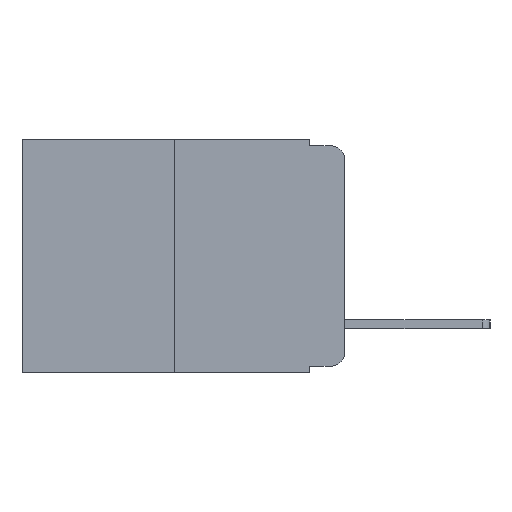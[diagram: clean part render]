
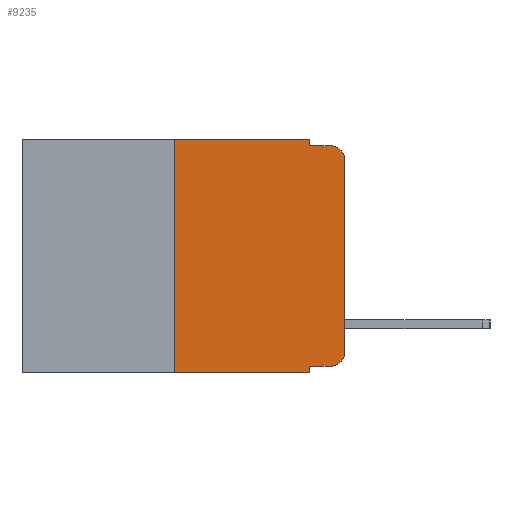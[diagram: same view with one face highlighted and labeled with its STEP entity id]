
A CAD part, left-side view. The second image highlights one B-rep face of the part: STEP entity #9235.
In plain terms, the highlighted planar face has unit normal (-1, 0, 0).
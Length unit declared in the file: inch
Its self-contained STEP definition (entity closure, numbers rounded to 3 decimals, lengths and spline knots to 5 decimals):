
#5 = VECTOR ( 'NONE', #6493, 39.37008 ) ;
#9 = EDGE_LOOP ( 'NONE', ( #9346, #6565, #7143, #6983, #9529, #5857, #39, #6434, #5657, #5868 ) ) ;
#39 = ORIENTED_EDGE ( 'NONE', *, *, #10191, .T. ) ;
#165 = VECTOR ( 'NONE', #2840, 39.37008 ) ;
#328 = LINE ( 'NONE', #6843, #5 ) ;
#520 = DIRECTION ( 'NONE',  ( 0., 0., 1. ) ) ;
#563 = VERTEX_POINT ( 'NONE', #4030 ) ;
#974 = VERTEX_POINT ( 'NONE', #6108 ) ;
#1439 = DIRECTION ( 'NONE',  ( -1., 0., 0. ) ) ;
#1712 = DIRECTION ( 'NONE',  ( 0., 0., -1. ) ) ;
#1723 = CARTESIAN_POINT ( 'NONE',  ( 0., 0.051, -0.333 ) ) ;
#1991 = VERTEX_POINT ( 'NONE', #8813 ) ;
#2165 = CARTESIAN_POINT ( 'NONE',  ( 0., 0., -0.03 ) ) ;
#2497 = CARTESIAN_POINT ( 'NONE',  ( 0., 0., -0.313 ) ) ;
#2683 = LINE ( 'NONE', #5300, #6839 ) ;
#2757 = VECTOR ( 'NONE', #11099, 39.37008 ) ;
#2840 = DIRECTION ( 'NONE',  ( 0., 0., 1. ) ) ;
#3433 = CARTESIAN_POINT ( 'NONE',  ( 0., 0.25, 0. ) ) ;
#3440 = DIRECTION ( 'NONE',  ( 0., -1., 0. ) ) ;
#3951 = VERTEX_POINT ( 'NONE', #2165 ) ;
#4030 = CARTESIAN_POINT ( 'NONE',  ( 0., 0.25, 0. ) ) ;
#4258 = EDGE_CURVE ( 'NONE', #974, #10230, #5118, .T. ) ;
#4303 = DIRECTION ( 'NONE',  ( 0., 0., -1. ) ) ;
#4307 = VERTEX_POINT ( 'NONE', #2497 ) ;
#4346 = FACE_OUTER_BOUND ( 'NONE', #9, .T. ) ;
#4767 = VERTEX_POINT ( 'NONE', #1723 ) ;
#4855 = VERTEX_POINT ( 'NONE', #11409 ) ;
#5091 = DIRECTION ( 'NONE',  ( 0., 0., -1. ) ) ;
#5118 = LINE ( 'NONE', #7505, #2757 ) ;
#5203 = VECTOR ( 'NONE', #3440, 39.37008 ) ;
#5300 = CARTESIAN_POINT ( 'NONE',  ( 0., 0.473, 0. ) ) ;
#5405 = EDGE_CURVE ( 'NONE', #1991, #974, #8115, .T. ) ;
#5516 = VERTEX_POINT ( 'NONE', #8456 ) ;
#5564 = DIRECTION ( 'NONE',  ( 0., 0., -1. ) ) ;
#5657 = ORIENTED_EDGE ( 'NONE', *, *, #7426, .T. ) ;
#5785 = VECTOR ( 'NONE', #5564, 39.37008 ) ;
#5857 = ORIENTED_EDGE ( 'NONE', *, *, #11788, .F. ) ;
#5868 = ORIENTED_EDGE ( 'NONE', *, *, #7997, .T. ) ;
#5904 = CARTESIAN_POINT ( 'NONE',  ( 0., 0.051, 0. ) ) ;
#5957 = VECTOR ( 'NONE', #520, 39.37008 ) ;
#6108 = CARTESIAN_POINT ( 'NONE',  ( 0., 0.051, -0.01 ) ) ;
#6434 = ORIENTED_EDGE ( 'NONE', *, *, #9062, .F. ) ;
#6493 = DIRECTION ( 'NONE',  ( 0., -1., 0. ) ) ;
#6565 = ORIENTED_EDGE ( 'NONE', *, *, #11217, .T. ) ;
#6824 = CARTESIAN_POINT ( 'NONE',  ( 0., 0.02, -0.03 ) ) ;
#6839 = VECTOR ( 'NONE', #8361, 39.37008 ) ;
#6843 = CARTESIAN_POINT ( 'NONE',  ( 0., 0.051, -0.333 ) ) ;
#6894 = DIRECTION ( 'NONE',  ( 1., 0., 0. ) ) ;
#6983 = ORIENTED_EDGE ( 'NONE', *, *, #5405, .F. ) ;
#7072 = CARTESIAN_POINT ( 'NONE',  ( 0., 0.051, 0. ) ) ;
#7143 = ORIENTED_EDGE ( 'NONE', *, *, #4258, .F. ) ;
#7426 = EDGE_CURVE ( 'NONE', #4767, #5516, #328, .T. ) ;
#7505 = CARTESIAN_POINT ( 'NONE',  ( 0., 0.051, -0.01 ) ) ;
#7689 = DIRECTION ( 'NONE',  ( 0., 0., -1. ) ) ;
#7997 = EDGE_CURVE ( 'NONE', #5516, #4307, #9570, .T. ) ;
#8025 = EDGE_CURVE ( 'NONE', #563, #1991, #2683, .T. ) ;
#8115 = LINE ( 'NONE', #5904, #5785 ) ;
#8126 = CARTESIAN_POINT ( 'NONE',  ( 0., 0., 0. ) ) ;
#8284 = LINE ( 'NONE', #3433, #5957 ) ;
#8361 = DIRECTION ( 'NONE',  ( 0., -1., 0. ) ) ;
#8421 = AXIS2_PLACEMENT_3D ( 'NONE', #8680, #6894, #4303 ) ;
#8448 = LINE ( 'NONE', #7072, #11033 ) ;
#8456 = CARTESIAN_POINT ( 'NONE',  ( 0., 0.02, -0.333 ) ) ;
#8680 = CARTESIAN_POINT ( 'NONE',  ( 0., 0.473, 0. ) ) ;
#8713 = CARTESIAN_POINT ( 'NONE',  ( 0., 0.473, -0.343 ) ) ;
#8813 = CARTESIAN_POINT ( 'NONE',  ( 0., 0.051, 0. ) ) ;
#9062 = EDGE_CURVE ( 'NONE', #4767, #10323, #8448, .T. ) ;
#9149 = DIRECTION ( 'NONE',  ( -1., 0., 0. ) ) ;
#9165 = CARTESIAN_POINT ( 'NONE',  ( 0., 0.02, -0.313 ) ) ;
#9235 = ADVANCED_FACE ( 'NONE', ( #4346 ), #9677, .F. ) ;
#9346 = ORIENTED_EDGE ( 'NONE', *, *, #10810, .T. ) ;
#9391 = AXIS2_PLACEMENT_3D ( 'NONE', #9165, #9149, #5091 ) ;
#9529 = ORIENTED_EDGE ( 'NONE', *, *, #8025, .F. ) ;
#9570 = CIRCLE ( 'NONE', #9391, 0.02 ) ;
#9677 = PLANE ( 'NONE',  #8421 ) ;
#9733 = LINE ( 'NONE', #8126, #165 ) ;
#9761 = LINE ( 'NONE', #8713, #5203 ) ;
#10191 = EDGE_CURVE ( 'NONE', #4855, #10323, #9761, .T. ) ;
#10230 = VERTEX_POINT ( 'NONE', #11692 ) ;
#10323 = VERTEX_POINT ( 'NONE', #11932 ) ;
#10810 = EDGE_CURVE ( 'NONE', #4307, #3951, #9733, .T. ) ;
#11033 = VECTOR ( 'NONE', #1712, 39.37008 ) ;
#11099 = DIRECTION ( 'NONE',  ( 0., -1., 0. ) ) ;
#11217 = EDGE_CURVE ( 'NONE', #3951, #10230, #11765, .T. ) ;
#11409 = CARTESIAN_POINT ( 'NONE',  ( 0., 0.25, -0.343 ) ) ;
#11639 = AXIS2_PLACEMENT_3D ( 'NONE', #6824, #1439, #7689 ) ;
#11692 = CARTESIAN_POINT ( 'NONE',  ( 0., 0.02, -0.01 ) ) ;
#11765 = CIRCLE ( 'NONE', #11639, 0.02 ) ;
#11788 = EDGE_CURVE ( 'NONE', #4855, #563, #8284, .T. ) ;
#11932 = CARTESIAN_POINT ( 'NONE',  ( 0., 0.051, -0.343 ) ) ;
